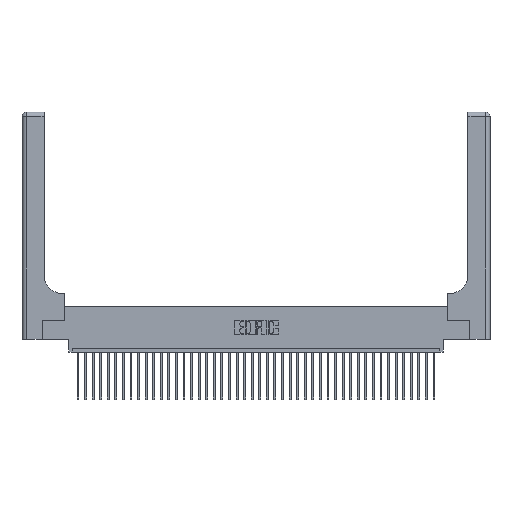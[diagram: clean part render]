
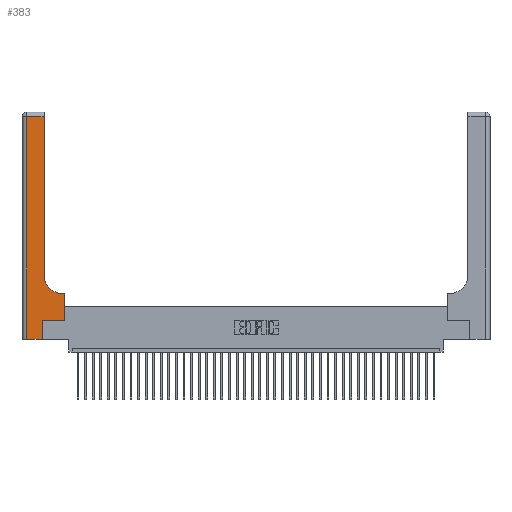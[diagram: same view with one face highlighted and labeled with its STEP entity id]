
A CAD part, top view. The second image highlights one B-rep face of the part: STEP entity #383.
In plain terms, the highlighted planar face has unit normal (0, 0, 1).
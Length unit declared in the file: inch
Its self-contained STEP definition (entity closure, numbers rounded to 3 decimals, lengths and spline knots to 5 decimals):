
#130 = VERTEX_POINT ( 'NONE', #37718 ) ;
#383 = ADVANCED_FACE ( 'NONE', ( #3967 ), #5648, .F. ) ;
#1206 = DIRECTION ( 'NONE',  ( 0., 0., -1. ) ) ;
#2086 = LINE ( 'NONE', #22752, #34446 ) ;
#2255 = EDGE_CURVE ( 'NONE', #23168, #24552, #40180, .T. ) ;
#2403 = VECTOR ( 'NONE', #36978, 39.37008 ) ;
#3161 = LINE ( 'NONE', #20360, #17938 ) ;
#3383 = ORIENTED_EDGE ( 'NONE', *, *, #20501, .T. ) ;
#3967 = FACE_OUTER_BOUND ( 'NONE', #34524, .T. ) ;
#4615 = LINE ( 'NONE', #10394, #14934 ) ;
#4978 = EDGE_CURVE ( 'NONE', #21930, #130, #19826, .T. ) ;
#5138 = ORIENTED_EDGE ( 'NONE', *, *, #4978, .T. ) ;
#5648 = PLANE ( 'NONE',  #38416 ) ;
#5781 = ORIENTED_EDGE ( 'NONE', *, *, #38409, .T. ) ;
#8269 = VERTEX_POINT ( 'NONE', #10190 ) ;
#8936 = CARTESIAN_POINT ( 'NONE',  ( 0., 3., 0.37 ) ) ;
#9000 = CARTESIAN_POINT ( 'NONE',  ( 0.5415, 0.6, 0.37 ) ) ;
#9249 = CARTESIAN_POINT ( 'NONE',  ( 0.06, 2.94, 0.37 ) ) ;
#9532 = LINE ( 'NONE', #19652, #25687 ) ;
#9758 = EDGE_CURVE ( 'NONE', #33602, #31952, #14470, .T. ) ;
#10190 = CARTESIAN_POINT ( 'NONE',  ( 0.5585, 0.25, 0.37 ) ) ;
#10394 = CARTESIAN_POINT ( 'NONE',  ( 0.5585, 0.25, 0.37 ) ) ;
#11029 = VECTOR ( 'NONE', #35894, 39.37008 ) ;
#13238 = CARTESIAN_POINT ( 'NONE',  ( 0.2915, 2.94, 0.37 ) ) ;
#13712 = DIRECTION ( 'NONE',  ( 0., 0., -1. ) ) ;
#13924 = DIRECTION ( 'NONE',  ( 0., -1., 0. ) ) ;
#13959 = ORIENTED_EDGE ( 'NONE', *, *, #38582, .T. ) ;
#14470 = LINE ( 'NONE', #31901, #11029 ) ;
#14934 = VECTOR ( 'NONE', #35491, 39.37008 ) ;
#15206 = CARTESIAN_POINT ( 'NONE',  ( 0.269, 0., 0.37 ) ) ;
#17091 = EDGE_CURVE ( 'NONE', #8269, #33602, #4615, .T. ) ;
#17144 = DIRECTION ( 'NONE',  ( -1., 0., 0. ) ) ;
#17938 = VECTOR ( 'NONE', #23914, 39.37008 ) ;
#18479 = CARTESIAN_POINT ( 'NONE',  ( 0.06, 0., 0.37 ) ) ;
#18659 = ORIENTED_EDGE ( 'NONE', *, *, #9758, .T. ) ;
#19540 = ORIENTED_EDGE ( 'NONE', *, *, #31076, .T. ) ;
#19652 = CARTESIAN_POINT ( 'NONE',  ( 0., 0., 0.37 ) ) ;
#19826 = LINE ( 'NONE', #15206, #21332 ) ;
#20064 = ORIENTED_EDGE ( 'NONE', *, *, #2255, .T. ) ;
#20360 = CARTESIAN_POINT ( 'NONE',  ( 0.269, 0.25, 0.37 ) ) ;
#20501 = EDGE_CURVE ( 'NONE', #24552, #30312, #2086, .T. ) ;
#21332 = VECTOR ( 'NONE', #34136, 39.37008 ) ;
#21808 = CARTESIAN_POINT ( 'NONE',  ( 0.2915, 0.85, 0.37 ) ) ;
#21930 = VERTEX_POINT ( 'NONE', #23545 ) ;
#22211 = ORIENTED_EDGE ( 'NONE', *, *, #38606, .T. ) ;
#22571 = CIRCLE ( 'NONE', #38220, 0.25 ) ;
#22752 = CARTESIAN_POINT ( 'NONE',  ( 0., 2.94, 0.37 ) ) ;
#23168 = VERTEX_POINT ( 'NONE', #21808 ) ;
#23545 = CARTESIAN_POINT ( 'NONE',  ( 0.269, 0., 0.37 ) ) ;
#23914 = DIRECTION ( 'NONE',  ( 1., 0., 0. ) ) ;
#24552 = VERTEX_POINT ( 'NONE', #13238 ) ;
#25687 = VECTOR ( 'NONE', #38274, 39.37008 ) ;
#26189 = CARTESIAN_POINT ( 'NONE',  ( 0.5415, 0.85, 0.37 ) ) ;
#28212 = VECTOR ( 'NONE', #13924, 39.37008 ) ;
#29660 = LINE ( 'NONE', #32673, #28212 ) ;
#30312 = VERTEX_POINT ( 'NONE', #9249 ) ;
#30427 = CARTESIAN_POINT ( 'NONE',  ( 0.2915, 3., 0.37 ) ) ;
#31076 = EDGE_CURVE ( 'NONE', #31952, #23168, #22571, .T. ) ;
#31901 = CARTESIAN_POINT ( 'NONE',  ( 0.2915, 0.6, 0.37 ) ) ;
#31952 = VERTEX_POINT ( 'NONE', #9000 ) ;
#32673 = CARTESIAN_POINT ( 'NONE',  ( 0.06, 3., 0.37 ) ) ;
#33291 = VERTEX_POINT ( 'NONE', #18479 ) ;
#33602 = VERTEX_POINT ( 'NONE', #36223 ) ;
#34136 = DIRECTION ( 'NONE',  ( 0., 1., 0. ) ) ;
#34446 = VECTOR ( 'NONE', #38234, 39.37008 ) ;
#34524 = EDGE_LOOP ( 'NONE', ( #20064, #3383, #13959, #5781, #5138, #22211, #36845, #18659, #19540 ) ) ;
#35491 = DIRECTION ( 'NONE',  ( 0., 1., 0. ) ) ;
#35894 = DIRECTION ( 'NONE',  ( -1., 0., 0. ) ) ;
#36223 = CARTESIAN_POINT ( 'NONE',  ( 0.5585, 0.6, 0.37 ) ) ;
#36845 = ORIENTED_EDGE ( 'NONE', *, *, #17091, .T. ) ;
#36978 = DIRECTION ( 'NONE',  ( 0., 1., 0. ) ) ;
#37718 = CARTESIAN_POINT ( 'NONE',  ( 0.269, 0.25, 0.37 ) ) ;
#38220 = AXIS2_PLACEMENT_3D ( 'NONE', #26189, #13712, #38507 ) ;
#38234 = DIRECTION ( 'NONE',  ( -1., 0., 0. ) ) ;
#38274 = DIRECTION ( 'NONE',  ( 1., 0., 0. ) ) ;
#38409 = EDGE_CURVE ( 'NONE', #33291, #21930, #9532, .T. ) ;
#38416 = AXIS2_PLACEMENT_3D ( 'NONE', #8936, #1206, #17144 ) ;
#38507 = DIRECTION ( 'NONE',  ( 1., 0., 0. ) ) ;
#38582 = EDGE_CURVE ( 'NONE', #30312, #33291, #29660, .T. ) ;
#38606 = EDGE_CURVE ( 'NONE', #130, #8269, #3161, .T. ) ;
#40180 = LINE ( 'NONE', #30427, #2403 ) ;
